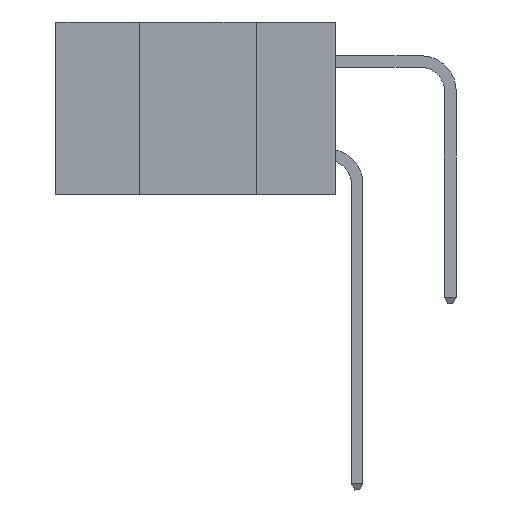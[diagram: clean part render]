
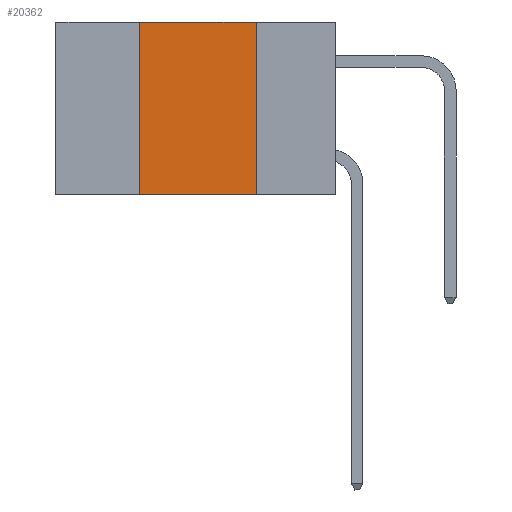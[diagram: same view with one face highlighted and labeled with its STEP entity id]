
A CAD part, left-side view. The second image highlights one B-rep face of the part: STEP entity #20362.
In plain terms, the highlighted planar face has unit normal (-1, 0, 0).
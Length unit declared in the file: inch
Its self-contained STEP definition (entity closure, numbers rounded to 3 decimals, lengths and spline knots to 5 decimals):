
#52 = CARTESIAN_POINT ( 'NONE',  ( 0., 0.17, 0. ) ) ;
#486 = VECTOR ( 'NONE', #27137, 39.37008 ) ;
#1422 = PLANE ( 'NONE',  #32338 ) ;
#2236 = CARTESIAN_POINT ( 'NONE',  ( 0., 0.6, -0.37 ) ) ;
#2251 = EDGE_CURVE ( 'NONE', #22847, #15898, #21698, .T. ) ;
#3084 = VECTOR ( 'NONE', #32230, 39.37008 ) ;
#4527 = CARTESIAN_POINT ( 'NONE',  ( 0., 0.17, -0.37 ) ) ;
#7427 = VECTOR ( 'NONE', #15923, 39.37008 ) ;
#8387 = CARTESIAN_POINT ( 'NONE',  ( 0., 0.42, 0. ) ) ;
#9728 = EDGE_CURVE ( 'NONE', #22847, #31699, #20889, .T. ) ;
#10429 = ORIENTED_EDGE ( 'NONE', *, *, #26238, .F. ) ;
#12687 = EDGE_CURVE ( 'NONE', #17168, #15898, #13597, .T. ) ;
#12898 = LINE ( 'NONE', #15225, #17272 ) ;
#12960 = CARTESIAN_POINT ( 'NONE',  ( 0., 0.17, 0. ) ) ;
#13597 = LINE ( 'NONE', #12960, #7427 ) ;
#15225 = CARTESIAN_POINT ( 'NONE',  ( 0., 0.6, 0. ) ) ;
#15388 = DIRECTION ( 'NONE',  ( 0., -1., 0. ) ) ;
#15611 = CARTESIAN_POINT ( 'NONE',  ( 0., 0.42, 0. ) ) ;
#15898 = VERTEX_POINT ( 'NONE', #4527 ) ;
#15923 = DIRECTION ( 'NONE',  ( 0., 0., -1. ) ) ;
#17168 = VERTEX_POINT ( 'NONE', #52 ) ;
#17272 = VECTOR ( 'NONE', #15388, 39.37008 ) ;
#18243 = CARTESIAN_POINT ( 'NONE',  ( 0., 0.42, -0.37 ) ) ;
#19080 = DIRECTION ( 'NONE',  ( 0., 0., -1. ) ) ;
#19565 = DIRECTION ( 'NONE',  ( 1., 0., 0. ) ) ;
#20362 = ADVANCED_FACE ( 'NONE', ( #32246 ), #1422, .F. ) ;
#20889 = LINE ( 'NONE', #8387, #3084 ) ;
#21698 = LINE ( 'NONE', #2236, #486 ) ;
#22474 = ORIENTED_EDGE ( 'NONE', *, *, #2251, .T. ) ;
#22847 = VERTEX_POINT ( 'NONE', #18243 ) ;
#24345 = CARTESIAN_POINT ( 'NONE',  ( 0., 0.6, 0. ) ) ;
#26238 = EDGE_CURVE ( 'NONE', #31699, #17168, #12898, .T. ) ;
#27137 = DIRECTION ( 'NONE',  ( 0., -1., 0. ) ) ;
#28202 = EDGE_LOOP ( 'NONE', ( #30374, #10429, #30428, #22474 ) ) ;
#30374 = ORIENTED_EDGE ( 'NONE', *, *, #12687, .F. ) ;
#30428 = ORIENTED_EDGE ( 'NONE', *, *, #9728, .F. ) ;
#31699 = VERTEX_POINT ( 'NONE', #15611 ) ;
#32230 = DIRECTION ( 'NONE',  ( 0., 0., 1. ) ) ;
#32246 = FACE_OUTER_BOUND ( 'NONE', #28202, .T. ) ;
#32338 = AXIS2_PLACEMENT_3D ( 'NONE', #24345, #19565, #19080 ) ;
